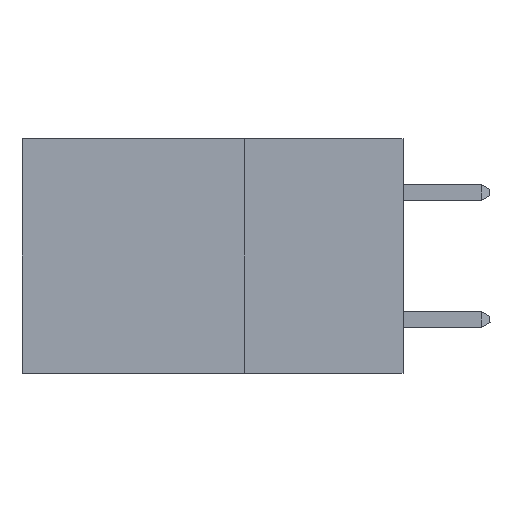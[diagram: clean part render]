
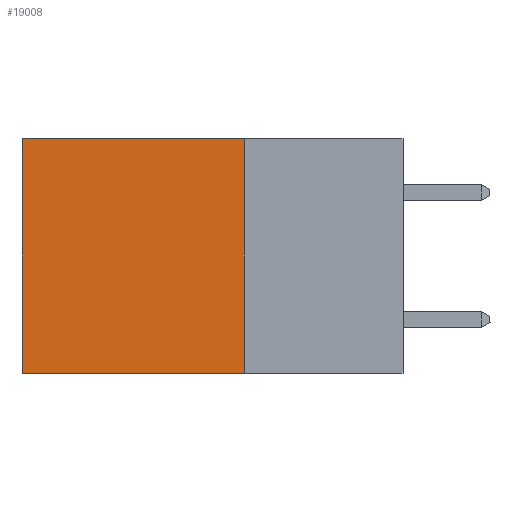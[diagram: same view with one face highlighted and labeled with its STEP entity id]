
A CAD part, left-side view. The second image highlights one B-rep face of the part: STEP entity #19008.
In plain terms, the highlighted planar face has unit normal (-1, 0, 0).
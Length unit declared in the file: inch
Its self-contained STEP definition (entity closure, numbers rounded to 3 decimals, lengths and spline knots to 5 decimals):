
#1102 = VECTOR ( 'NONE', #33148, 39.37008 ) ;
#1713 = LINE ( 'NONE', #36013, #19468 ) ;
#4053 = VERTEX_POINT ( 'NONE', #27071 ) ;
#4103 = VECTOR ( 'NONE', #16240, 39.37008 ) ;
#4345 = DIRECTION ( 'NONE',  ( 0., 1., 0. ) ) ;
#4898 = DIRECTION ( 'NONE',  ( 0., 1., 0. ) ) ;
#5046 = CARTESIAN_POINT ( 'NONE',  ( 0.2875, 0.6, 0. ) ) ;
#6043 = VERTEX_POINT ( 'NONE', #21692 ) ;
#6152 = CARTESIAN_POINT ( 'NONE',  ( 0.2875, 0.25, -0.37 ) ) ;
#7570 = CARTESIAN_POINT ( 'NONE',  ( 0.2875, 0.25, 0. ) ) ;
#8514 = EDGE_CURVE ( 'NONE', #4053, #17742, #12486, .T. ) ;
#8857 = EDGE_CURVE ( 'NONE', #6043, #9680, #29183, .T. ) ;
#9585 = CARTESIAN_POINT ( 'NONE',  ( 0.2875, 0.6, -0.37 ) ) ;
#9680 = VERTEX_POINT ( 'NONE', #9585 ) ;
#9977 = AXIS2_PLACEMENT_3D ( 'NONE', #7570, #23172, #17109 ) ;
#10889 = ORIENTED_EDGE ( 'NONE', *, *, #8514, .F. ) ;
#12486 = LINE ( 'NONE', #25442, #4103 ) ;
#15017 = EDGE_CURVE ( 'NONE', #4053, #6043, #1713, .T. ) ;
#15844 = ORIENTED_EDGE ( 'NONE', *, *, #15017, .T. ) ;
#16240 = DIRECTION ( 'NONE',  ( 0., 0., -1. ) ) ;
#17109 = DIRECTION ( 'NONE',  ( 0., 0., -1. ) ) ;
#17243 = PLANE ( 'NONE',  #9977 ) ;
#17742 = VERTEX_POINT ( 'NONE', #6152 ) ;
#19008 = ADVANCED_FACE ( 'NONE', ( #35340 ), #17243, .F. ) ;
#19468 = VECTOR ( 'NONE', #4898, 39.37008 ) ;
#19503 = CARTESIAN_POINT ( 'NONE',  ( 0.2875, 0.25, -0.37 ) ) ;
#21692 = CARTESIAN_POINT ( 'NONE',  ( 0.2875, 0.6, 0. ) ) ;
#22491 = EDGE_CURVE ( 'NONE', #17742, #9680, #24999, .T. ) ;
#23172 = DIRECTION ( 'NONE',  ( 1., 0., 0. ) ) ;
#23345 = ORIENTED_EDGE ( 'NONE', *, *, #8857, .T. ) ;
#24999 = LINE ( 'NONE', #19503, #32394 ) ;
#25442 = CARTESIAN_POINT ( 'NONE',  ( 0.2875, 0.25, 0. ) ) ;
#27071 = CARTESIAN_POINT ( 'NONE',  ( 0.2875, 0.25, 0. ) ) ;
#29183 = LINE ( 'NONE', #5046, #1102 ) ;
#32394 = VECTOR ( 'NONE', #4345, 39.37008 ) ;
#33148 = DIRECTION ( 'NONE',  ( 0., 0., -1. ) ) ;
#35340 = FACE_OUTER_BOUND ( 'NONE', #40242, .T. ) ;
#36013 = CARTESIAN_POINT ( 'NONE',  ( 0.2875, 0.25, 0. ) ) ;
#40242 = EDGE_LOOP ( 'NONE', ( #23345, #40380, #10889, #15844 ) ) ;
#40380 = ORIENTED_EDGE ( 'NONE', *, *, #22491, .F. ) ;
